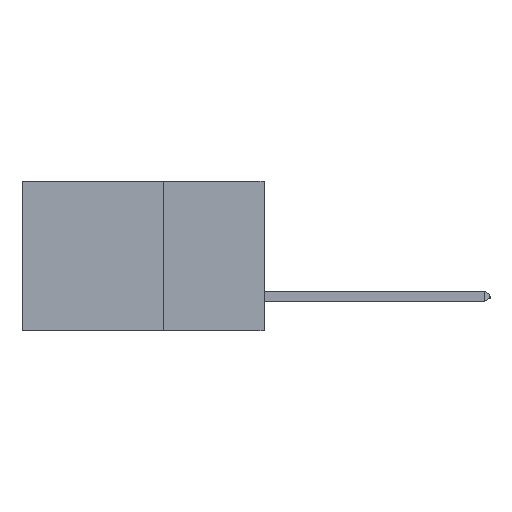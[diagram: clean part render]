
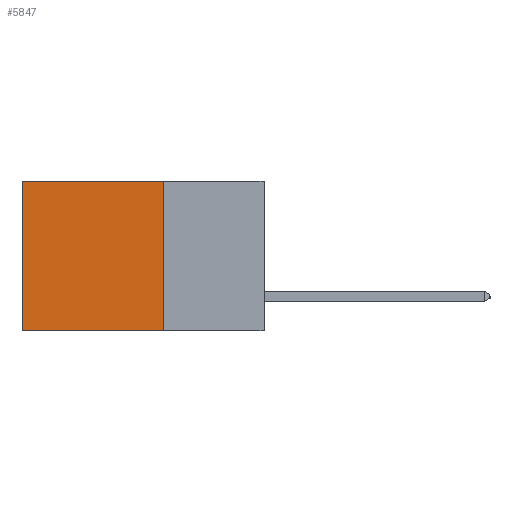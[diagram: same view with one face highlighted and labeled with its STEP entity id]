
A CAD part, left-side view. The second image highlights one B-rep face of the part: STEP entity #5847.
In plain terms, the highlighted planar face has unit normal (-1, 0, 0).
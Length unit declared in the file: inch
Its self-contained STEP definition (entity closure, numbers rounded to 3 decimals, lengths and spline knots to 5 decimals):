
#342 = ORIENTED_EDGE ( 'NONE', *, *, #14975, .F. ) ;
#613 = CARTESIAN_POINT ( 'NONE',  ( 0.298, 0.6, 0. ) ) ;
#1462 = PLANE ( 'NONE',  #24396 ) ;
#1812 = VECTOR ( 'NONE', #2706, 39.37008 ) ;
#1839 = LINE ( 'NONE', #3475, #11855 ) ;
#2571 = VERTEX_POINT ( 'NONE', #3709 ) ;
#2659 = VECTOR ( 'NONE', #2862, 39.37008 ) ;
#2706 = DIRECTION ( 'NONE',  ( 0., 0., -1. ) ) ;
#2862 = DIRECTION ( 'NONE',  ( 0., 0., -1. ) ) ;
#2974 = EDGE_CURVE ( 'NONE', #15877, #2571, #19630, .T. ) ;
#3475 = CARTESIAN_POINT ( 'NONE',  ( 0.298, 0.25, -0.37 ) ) ;
#3603 = DIRECTION ( 'NONE',  ( 0., 0., -1. ) ) ;
#3709 = CARTESIAN_POINT ( 'NONE',  ( 0.298, 0.6, -0.37 ) ) ;
#5156 = FACE_OUTER_BOUND ( 'NONE', #25854, .T. ) ;
#5669 = EDGE_CURVE ( 'NONE', #9359, #15877, #9827, .T. ) ;
#5847 = ADVANCED_FACE ( 'NONE', ( #5156 ), #1462, .F. ) ;
#7452 = VERTEX_POINT ( 'NONE', #19430 ) ;
#9305 = CARTESIAN_POINT ( 'NONE',  ( 0.298, 0.25, 0. ) ) ;
#9359 = VERTEX_POINT ( 'NONE', #24839 ) ;
#9827 = LINE ( 'NONE', #9305, #20454 ) ;
#9899 = DIRECTION ( 'NONE',  ( 0., 1., 0. ) ) ;
#11855 = VECTOR ( 'NONE', #9899, 39.37008 ) ;
#14220 = CARTESIAN_POINT ( 'NONE',  ( 0.298, 0.25, 0. ) ) ;
#14975 = EDGE_CURVE ( 'NONE', #7452, #2571, #1839, .T. ) ;
#15381 = EDGE_CURVE ( 'NONE', #9359, #7452, #18141, .T. ) ;
#15471 = CARTESIAN_POINT ( 'NONE',  ( 0.298, 0.25, 0. ) ) ;
#15877 = VERTEX_POINT ( 'NONE', #23419 ) ;
#16371 = DIRECTION ( 'NONE',  ( 1., 0., 0. ) ) ;
#16588 = ORIENTED_EDGE ( 'NONE', *, *, #5669, .T. ) ;
#18141 = LINE ( 'NONE', #15471, #1812 ) ;
#19430 = CARTESIAN_POINT ( 'NONE',  ( 0.298, 0.25, -0.37 ) ) ;
#19630 = LINE ( 'NONE', #613, #2659 ) ;
#20454 = VECTOR ( 'NONE', #26368, 39.37008 ) ;
#21980 = ORIENTED_EDGE ( 'NONE', *, *, #2974, .T. ) ;
#23419 = CARTESIAN_POINT ( 'NONE',  ( 0.298, 0.6, 0. ) ) ;
#24396 = AXIS2_PLACEMENT_3D ( 'NONE', #14220, #16371, #3603 ) ;
#24684 = ORIENTED_EDGE ( 'NONE', *, *, #15381, .F. ) ;
#24839 = CARTESIAN_POINT ( 'NONE',  ( 0.298, 0.25, 0. ) ) ;
#25854 = EDGE_LOOP ( 'NONE', ( #21980, #342, #24684, #16588 ) ) ;
#26368 = DIRECTION ( 'NONE',  ( 0., 1., 0. ) ) ;
